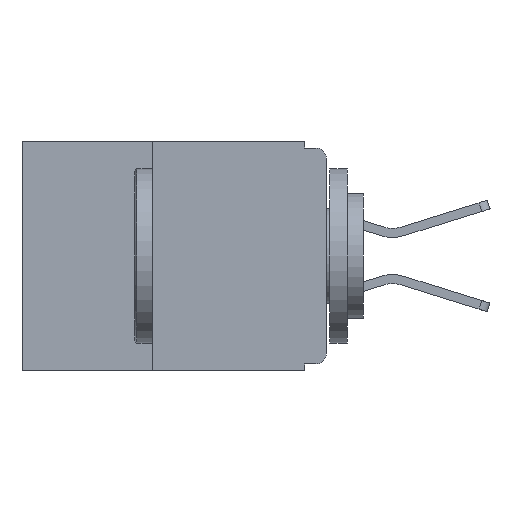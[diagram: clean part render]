
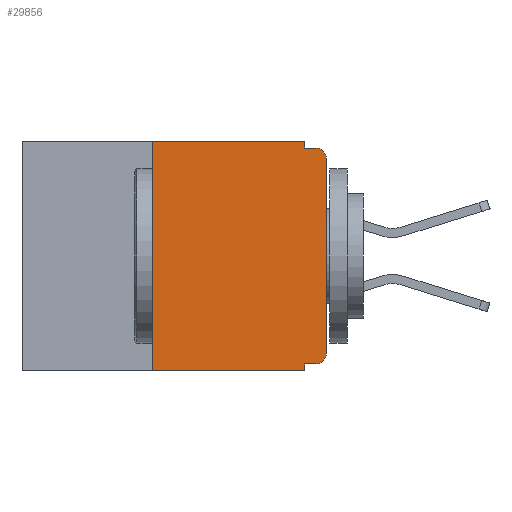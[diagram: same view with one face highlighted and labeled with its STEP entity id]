
A CAD part, left-side view. The second image highlights one B-rep face of the part: STEP entity #29856.
In plain terms, the highlighted planar face has unit normal (-1, 0, 0).
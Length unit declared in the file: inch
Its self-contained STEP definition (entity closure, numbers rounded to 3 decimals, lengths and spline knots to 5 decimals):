
#21 = DIRECTION ( 'NONE',  ( 0., 1., 0. ) ) ;
#351 = ORIENTED_EDGE ( 'NONE', *, *, #24436, .F. ) ;
#695 = CARTESIAN_POINT ( 'NONE',  ( 0., 0., -0.32 ) ) ;
#712 = ORIENTED_EDGE ( 'NONE', *, *, #34815, .F. ) ;
#849 = ORIENTED_EDGE ( 'NONE', *, *, #17266, .F. ) ;
#914 = ORIENTED_EDGE ( 'NONE', *, *, #15468, .T. ) ;
#979 = CARTESIAN_POINT ( 'NONE',  ( 0., 0.031, -0.01 ) ) ;
#1279 = ORIENTED_EDGE ( 'NONE', *, *, #4611, .F. ) ;
#1339 = CARTESIAN_POINT ( 'NONE',  ( 0., 0., -0.025 ) ) ;
#1369 = ORIENTED_EDGE ( 'NONE', *, *, #6440, .F. ) ;
#1505 = ORIENTED_EDGE ( 'NONE', *, *, #19779, .T. ) ;
#1556 = VECTOR ( 'NONE', #9865, 39.37008 ) ;
#2123 = AXIS2_PLACEMENT_3D ( 'NONE', #10474, #29313, #13228 ) ;
#2488 = VERTEX_POINT ( 'NONE', #8700 ) ;
#2712 = VERTEX_POINT ( 'NONE', #26611 ) ;
#4156 = VERTEX_POINT ( 'NONE', #979 ) ;
#4483 = DIRECTION ( 'NONE',  ( 0., 0., -1. ) ) ;
#4611 = EDGE_CURVE ( 'NONE', #2712, #34607, #23323, .T. ) ;
#4903 = CARTESIAN_POINT ( 'NONE',  ( 0., 0.015, -0.025 ) ) ;
#5342 = LINE ( 'NONE', #11290, #25973 ) ;
#5497 = VECTOR ( 'NONE', #21, 39.37008 ) ;
#6440 = EDGE_CURVE ( 'NONE', #19213, #2712, #26986, .T. ) ;
#6736 = CARTESIAN_POINT ( 'NONE',  ( 0., 0.437, 0. ) ) ;
#7147 = CARTESIAN_POINT ( 'NONE',  ( 0., 0., -0.01 ) ) ;
#7595 = DIRECTION ( 'NONE',  ( 0., 0., -1. ) ) ;
#8411 = AXIS2_PLACEMENT_3D ( 'NONE', #25902, #20665, #4483 ) ;
#8700 = CARTESIAN_POINT ( 'NONE',  ( 0., 0.031, 0. ) ) ;
#9148 = CARTESIAN_POINT ( 'NONE',  ( 0., 0.437, -0.33 ) ) ;
#9790 = CARTESIAN_POINT ( 'NONE',  ( 0., 0., 0. ) ) ;
#9865 = DIRECTION ( 'NONE',  ( 0., -1., 0. ) ) ;
#10474 = CARTESIAN_POINT ( 'NONE',  ( 0., 0.015, -0.305 ) ) ;
#11290 = CARTESIAN_POINT ( 'NONE',  ( 0., 0.25, -0.33 ) ) ;
#11924 = VECTOR ( 'NONE', #22906, 39.37008 ) ;
#12148 = VERTEX_POINT ( 'NONE', #18538 ) ;
#12476 = CIRCLE ( 'NONE', #24419, 0.015 ) ;
#12925 = VERTEX_POINT ( 'NONE', #1339 ) ;
#13028 = EDGE_CURVE ( 'NONE', #16101, #12925, #18693, .T. ) ;
#13228 = DIRECTION ( 'NONE',  ( 0., 0., -1. ) ) ;
#15239 = PLANE ( 'NONE',  #8411 ) ;
#15468 = EDGE_CURVE ( 'NONE', #15727, #34607, #32749, .T. ) ;
#15727 = VERTEX_POINT ( 'NONE', #26349 ) ;
#15912 = LINE ( 'NONE', #25887, #29356 ) ;
#16101 = VERTEX_POINT ( 'NONE', #28216 ) ;
#16198 = CARTESIAN_POINT ( 'NONE',  ( 0., 0.015, -0.32 ) ) ;
#17266 = EDGE_CURVE ( 'NONE', #15727, #12148, #5342, .T. ) ;
#18261 = LINE ( 'NONE', #6736, #11924 ) ;
#18538 = CARTESIAN_POINT ( 'NONE',  ( 0., 0.25, 0. ) ) ;
#18693 = LINE ( 'NONE', #9790, #31281 ) ;
#19213 = VERTEX_POINT ( 'NONE', #16198 ) ;
#19779 = EDGE_CURVE ( 'NONE', #19213, #16101, #24518, .T. ) ;
#20665 = DIRECTION ( 'NONE',  ( 1., 0., 0. ) ) ;
#22906 = DIRECTION ( 'NONE',  ( 0., -1., 0. ) ) ;
#23323 = LINE ( 'NONE', #32432, #30466 ) ;
#23739 = DIRECTION ( 'NONE',  ( -1., 0., 0. ) ) ;
#24419 = AXIS2_PLACEMENT_3D ( 'NONE', #4903, #23739, #7595 ) ;
#24436 = EDGE_CURVE ( 'NONE', #2488, #4156, #15912, .T. ) ;
#24488 = EDGE_CURVE ( 'NONE', #4156, #34507, #30182, .T. ) ;
#24518 = CIRCLE ( 'NONE', #2123, 0.015 ) ;
#24648 = CARTESIAN_POINT ( 'NONE',  ( 0., 0.031, -0.33 ) ) ;
#24773 = VECTOR ( 'NONE', #30704, 39.37008 ) ;
#25887 = CARTESIAN_POINT ( 'NONE',  ( 0., 0.031, 0. ) ) ;
#25902 = CARTESIAN_POINT ( 'NONE',  ( 0., 0.437, 0. ) ) ;
#25973 = VECTOR ( 'NONE', #30105, 39.37008 ) ;
#26349 = CARTESIAN_POINT ( 'NONE',  ( 0., 0.25, -0.33 ) ) ;
#26611 = CARTESIAN_POINT ( 'NONE',  ( 0., 0.031, -0.32 ) ) ;
#26986 = LINE ( 'NONE', #695, #5497 ) ;
#28216 = CARTESIAN_POINT ( 'NONE',  ( 0., 0., -0.305 ) ) ;
#28650 = DIRECTION ( 'NONE',  ( 0., 0., 1. ) ) ;
#28775 = EDGE_CURVE ( 'NONE', #12925, #34507, #12476, .T. ) ;
#29313 = DIRECTION ( 'NONE',  ( -1., 0., 0. ) ) ;
#29356 = VECTOR ( 'NONE', #31280, 39.37008 ) ;
#29593 = ORIENTED_EDGE ( 'NONE', *, *, #13028, .T. ) ;
#29856 = ADVANCED_FACE ( 'NONE', ( #33407 ), #15239, .F. ) ;
#30105 = DIRECTION ( 'NONE',  ( 0., 0., 1. ) ) ;
#30182 = LINE ( 'NONE', #7147, #1556 ) ;
#30466 = VECTOR ( 'NONE', #32503, 39.37008 ) ;
#30704 = DIRECTION ( 'NONE',  ( 0., -1., 0. ) ) ;
#31280 = DIRECTION ( 'NONE',  ( 0., 0., -1. ) ) ;
#31281 = VECTOR ( 'NONE', #28650, 39.37008 ) ;
#31607 = ORIENTED_EDGE ( 'NONE', *, *, #28775, .T. ) ;
#32099 = ORIENTED_EDGE ( 'NONE', *, *, #24488, .F. ) ;
#32300 = CARTESIAN_POINT ( 'NONE',  ( 0., 0.015, -0.01 ) ) ;
#32432 = CARTESIAN_POINT ( 'NONE',  ( 0., 0.031, -0.33 ) ) ;
#32503 = DIRECTION ( 'NONE',  ( 0., 0., -1. ) ) ;
#32749 = LINE ( 'NONE', #9148, #24773 ) ;
#33407 = FACE_OUTER_BOUND ( 'NONE', #34397, .T. ) ;
#34397 = EDGE_LOOP ( 'NONE', ( #29593, #31607, #32099, #351, #712, #849, #914, #1279, #1369, #1505 ) ) ;
#34507 = VERTEX_POINT ( 'NONE', #32300 ) ;
#34607 = VERTEX_POINT ( 'NONE', #24648 ) ;
#34815 = EDGE_CURVE ( 'NONE', #12148, #2488, #18261, .T. ) ;
